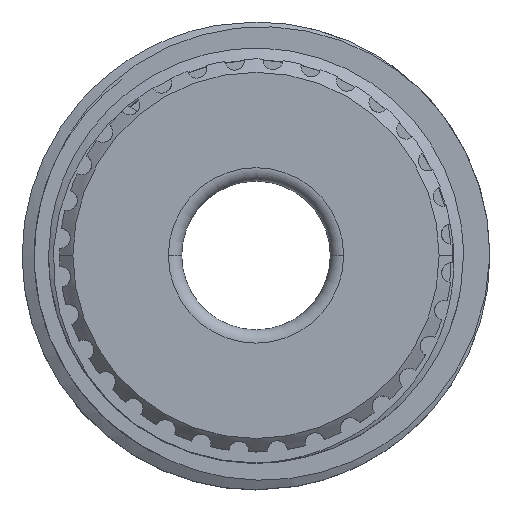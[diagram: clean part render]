
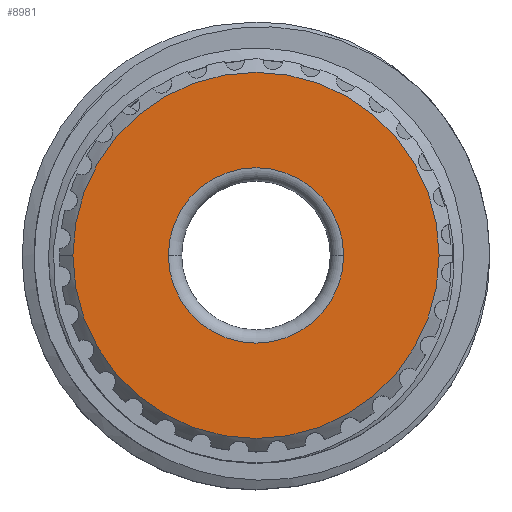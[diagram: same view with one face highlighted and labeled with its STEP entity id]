
A CAD part, top view. The second image highlights one B-rep face of the part: STEP entity #8981.
In plain terms, the highlighted planar face has unit normal (0, 0, 1).
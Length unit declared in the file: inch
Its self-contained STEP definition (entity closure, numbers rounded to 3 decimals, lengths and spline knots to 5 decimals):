
#564 = CARTESIAN_POINT ( 'NONE',  ( 0.328, 0., 1.46923 ) ) ;
#639 = CIRCLE ( 'NONE', #1616, 0.328 ) ;
#903 = CARTESIAN_POINT ( 'NONE',  ( 0.685, 0., 1.46923 ) ) ;
#939 = CARTESIAN_POINT ( 'NONE',  ( 0., 0., 1.46923 ) ) ;
#1297 = VERTEX_POINT ( 'NONE', #4392 ) ;
#1501 = EDGE_CURVE ( 'NONE', #10331, #6040, #639, .T. ) ;
#1510 = FACE_BOUND ( 'NONE', #5442, .T. ) ;
#1616 = AXIS2_PLACEMENT_3D ( 'NONE', #4649, #5852, #11811 ) ;
#1741 = DIRECTION ( 'NONE',  ( 0., 0., 1. ) ) ;
#2722 = AXIS2_PLACEMENT_3D ( 'NONE', #3720, #7672, #4741 ) ;
#3668 = ORIENTED_EDGE ( 'NONE', *, *, #7414, .T. ) ;
#3673 = CARTESIAN_POINT ( 'NONE',  ( -0.328, 0., 1.46923 ) ) ;
#3720 = CARTESIAN_POINT ( 'NONE',  ( 0., 0., 1.46923 ) ) ;
#3741 = DIRECTION ( 'NONE',  ( 0., 0., 1. ) ) ;
#3742 = VERTEX_POINT ( 'NONE', #903 ) ;
#3792 = PLANE ( 'NONE',  #9018 ) ;
#4344 = ORIENTED_EDGE ( 'NONE', *, *, #1501, .T. ) ;
#4392 = CARTESIAN_POINT ( 'NONE',  ( -0.685, 0., 1.46923 ) ) ;
#4649 = CARTESIAN_POINT ( 'NONE',  ( 0., 0., 1.46923 ) ) ;
#4741 = DIRECTION ( 'NONE',  ( 1., 0., 0. ) ) ;
#4767 = DIRECTION ( 'NONE',  ( 1., 0., 0. ) ) ;
#5442 = EDGE_LOOP ( 'NONE', ( #5940, #4344 ) ) ;
#5852 = DIRECTION ( 'NONE',  ( 0., 0., -1. ) ) ;
#5940 = ORIENTED_EDGE ( 'NONE', *, *, #9190, .T. ) ;
#6040 = VERTEX_POINT ( 'NONE', #564 ) ;
#6317 = CIRCLE ( 'NONE', #2722, 0.685 ) ;
#6746 = EDGE_CURVE ( 'NONE', #3742, #1297, #11562, .T. ) ;
#7414 = EDGE_CURVE ( 'NONE', #1297, #3742, #6317, .T. ) ;
#7672 = DIRECTION ( 'NONE',  ( 0., 0., 1. ) ) ;
#7791 = CARTESIAN_POINT ( 'NONE',  ( 0., 0., 1.46923 ) ) ;
#8981 = ADVANCED_FACE ( 'NONE', ( #1510, #9294 ), #3792, .T. ) ;
#9018 = AXIS2_PLACEMENT_3D ( 'NONE', #7791, #1741, #10899 ) ;
#9190 = EDGE_CURVE ( 'NONE', #6040, #10331, #10086, .T. ) ;
#9294 = FACE_OUTER_BOUND ( 'NONE', #12909, .T. ) ;
#10086 = CIRCLE ( 'NONE', #12698, 0.328 ) ;
#10331 = VERTEX_POINT ( 'NONE', #3673 ) ;
#10899 = DIRECTION ( 'NONE',  ( 1., 0., 0. ) ) ;
#10975 = CARTESIAN_POINT ( 'NONE',  ( 0., 0., 1.46923 ) ) ;
#11105 = DIRECTION ( 'NONE',  ( 1., 0., 0. ) ) ;
#11562 = CIRCLE ( 'NONE', #13026, 0.685 ) ;
#11811 = DIRECTION ( 'NONE',  ( 1., 0., 0. ) ) ;
#12016 = DIRECTION ( 'NONE',  ( 0., 0., -1. ) ) ;
#12608 = ORIENTED_EDGE ( 'NONE', *, *, #6746, .T. ) ;
#12698 = AXIS2_PLACEMENT_3D ( 'NONE', #939, #12016, #11105 ) ;
#12909 = EDGE_LOOP ( 'NONE', ( #3668, #12608 ) ) ;
#13026 = AXIS2_PLACEMENT_3D ( 'NONE', #10975, #3741, #4767 ) ;
